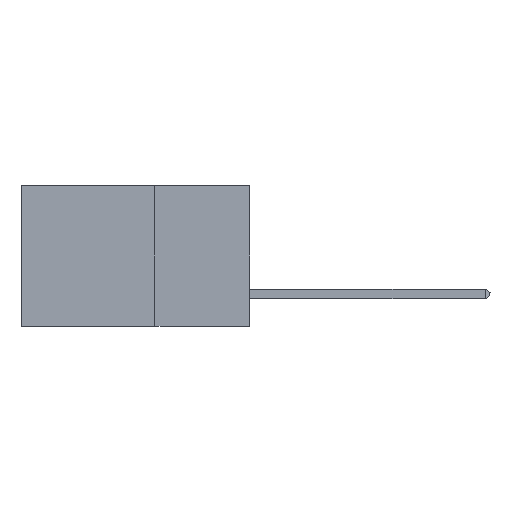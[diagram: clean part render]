
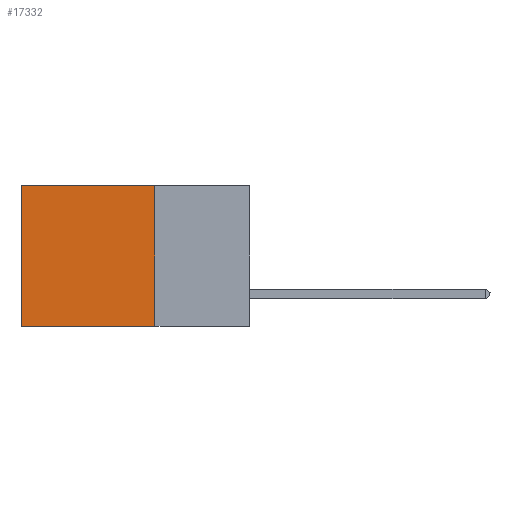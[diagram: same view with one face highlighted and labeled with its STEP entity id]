
A CAD part, left-side view. The second image highlights one B-rep face of the part: STEP entity #17332.
In plain terms, the highlighted planar face has unit normal (-1, 0, 0).
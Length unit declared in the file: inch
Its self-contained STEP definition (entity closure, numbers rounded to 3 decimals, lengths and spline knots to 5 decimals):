
#521 = DIRECTION ( 'NONE',  ( 0., 1., 0. ) ) ;
#3969 = CARTESIAN_POINT ( 'NONE',  ( 0.2875, 0.25, -0.37 ) ) ;
#4516 = CARTESIAN_POINT ( 'NONE',  ( 0.2875, 0.6, 0. ) ) ;
#4637 = CARTESIAN_POINT ( 'NONE',  ( 0.2875, 0.6, 0. ) ) ;
#6171 = VERTEX_POINT ( 'NONE', #16907 ) ;
#8434 = LINE ( 'NONE', #3969, #22150 ) ;
#9168 = VERTEX_POINT ( 'NONE', #35110 ) ;
#10865 = VECTOR ( 'NONE', #13736, 39.37008 ) ;
#13736 = DIRECTION ( 'NONE',  ( 0., 0., -1. ) ) ;
#14395 = DIRECTION ( 'NONE',  ( 0., 1., 0. ) ) ;
#16093 = ORIENTED_EDGE ( 'NONE', *, *, #24548, .T. ) ;
#16907 = CARTESIAN_POINT ( 'NONE',  ( 0.2875, 0.25, 0. ) ) ;
#17332 = ADVANCED_FACE ( 'NONE', ( #38092 ), #38865, .F. ) ;
#17911 = DIRECTION ( 'NONE',  ( 1., 0., 0. ) ) ;
#17975 = AXIS2_PLACEMENT_3D ( 'NONE', #36061, #17911, #29495 ) ;
#20620 = EDGE_CURVE ( 'NONE', #31191, #9168, #8434, .T. ) ;
#22150 = VECTOR ( 'NONE', #521, 39.37008 ) ;
#23370 = CARTESIAN_POINT ( 'NONE',  ( 0.2875, 0.25, 0. ) ) ;
#24342 = ORIENTED_EDGE ( 'NONE', *, *, #20620, .F. ) ;
#24425 = CARTESIAN_POINT ( 'NONE',  ( 0.2875, 0.25, -0.37 ) ) ;
#24548 = EDGE_CURVE ( 'NONE', #6171, #25563, #24653, .T. ) ;
#24653 = LINE ( 'NONE', #29661, #30286 ) ;
#25563 = VERTEX_POINT ( 'NONE', #4637 ) ;
#25730 = EDGE_CURVE ( 'NONE', #6171, #31191, #27352, .T. ) ;
#25967 = ORIENTED_EDGE ( 'NONE', *, *, #25730, .F. ) ;
#27352 = LINE ( 'NONE', #23370, #28722 ) ;
#28083 = EDGE_LOOP ( 'NONE', ( #35230, #24342, #25967, #16093 ) ) ;
#28722 = VECTOR ( 'NONE', #31850, 39.37008 ) ;
#29495 = DIRECTION ( 'NONE',  ( 0., 0., -1. ) ) ;
#29661 = CARTESIAN_POINT ( 'NONE',  ( 0.2875, 0.25, 0. ) ) ;
#30206 = LINE ( 'NONE', #4516, #10865 ) ;
#30286 = VECTOR ( 'NONE', #14395, 39.37008 ) ;
#31191 = VERTEX_POINT ( 'NONE', #24425 ) ;
#31850 = DIRECTION ( 'NONE',  ( 0., 0., -1. ) ) ;
#35110 = CARTESIAN_POINT ( 'NONE',  ( 0.2875, 0.6, -0.37 ) ) ;
#35230 = ORIENTED_EDGE ( 'NONE', *, *, #37179, .T. ) ;
#36061 = CARTESIAN_POINT ( 'NONE',  ( 0.2875, 0.25, 0. ) ) ;
#37179 = EDGE_CURVE ( 'NONE', #25563, #9168, #30206, .T. ) ;
#38092 = FACE_OUTER_BOUND ( 'NONE', #28083, .T. ) ;
#38865 = PLANE ( 'NONE',  #17975 ) ;
